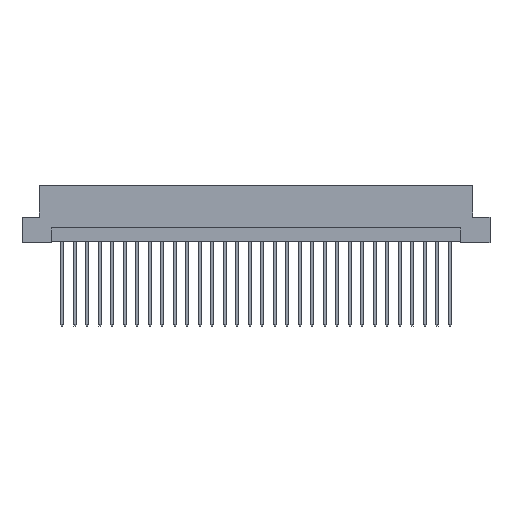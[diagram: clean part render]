
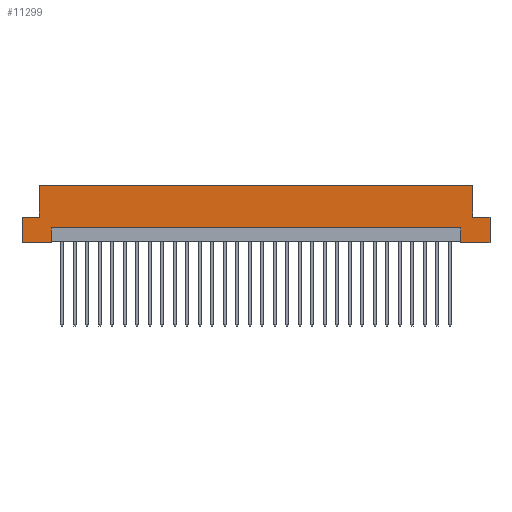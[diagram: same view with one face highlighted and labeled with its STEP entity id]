
A CAD part, front view. The second image highlights one B-rep face of the part: STEP entity #11299.
In plain terms, the highlighted planar face has unit normal (0, -1, 0).
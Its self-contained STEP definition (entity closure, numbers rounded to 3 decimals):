
#121 = VECTOR ( 'NONE', #6908, 1000. ) ;
#229 = VECTOR ( 'NONE', #6112, 1000. ) ;
#301 = DIRECTION ( 'NONE',  ( 0., 0., 1. ) ) ;
#396 = PLANE ( 'NONE',  #6061 ) ;
#691 = VERTEX_POINT ( 'NONE', #4877 ) ;
#767 = EDGE_CURVE ( 'NONE', #8356, #807, #3832, .T. ) ;
#798 = VECTOR ( 'NONE', #301, 1000. ) ;
#807 = VERTEX_POINT ( 'NONE', #4809 ) ;
#852 = CARTESIAN_POINT ( 'NONE',  ( -47.5, -4.3, 5.2 ) ) ;
#909 = CARTESIAN_POINT ( 'NONE',  ( -41.6, -4.3, 3. ) ) ;
#943 = ORIENTED_EDGE ( 'NONE', *, *, #10536, .T. ) ;
#1155 = CARTESIAN_POINT ( 'NONE',  ( 47.5, -4.3, 0. ) ) ;
#1309 = CARTESIAN_POINT ( 'NONE',  ( -47.5, -4.3, 0. ) ) ;
#1607 = LINE ( 'NONE', #7009, #10661 ) ;
#1705 = LINE ( 'NONE', #852, #11275 ) ;
#1811 = VERTEX_POINT ( 'NONE', #9847 ) ;
#1927 = DIRECTION ( 'NONE',  ( 1., 0., 0. ) ) ;
#2198 = LINE ( 'NONE', #10871, #5237 ) ;
#2203 = EDGE_CURVE ( 'NONE', #7240, #10167, #6225, .T. ) ;
#2415 = DIRECTION ( 'NONE',  ( 0., 1., 0. ) ) ;
#2458 = ORIENTED_EDGE ( 'NONE', *, *, #5085, .F. ) ;
#2568 = VERTEX_POINT ( 'NONE', #1309 ) ;
#2611 = CARTESIAN_POINT ( 'NONE',  ( -41.6, -4.3, 3. ) ) ;
#2728 = DIRECTION ( 'NONE',  ( 0., 0., -1. ) ) ;
#2834 = LINE ( 'NONE', #8767, #10973 ) ;
#2902 = ORIENTED_EDGE ( 'NONE', *, *, #3012, .F. ) ;
#2977 = VERTEX_POINT ( 'NONE', #5133 ) ;
#3012 = EDGE_CURVE ( 'NONE', #6895, #807, #11004, .T. ) ;
#3179 = DIRECTION ( 'NONE',  ( 1., 0., 0. ) ) ;
#3257 = CARTESIAN_POINT ( 'NONE',  ( 41.6, -4.3, 0. ) ) ;
#3782 = LINE ( 'NONE', #6784, #9607 ) ;
#3831 = CARTESIAN_POINT ( 'NONE',  ( -47.5, -4.3, 11.6 ) ) ;
#3832 = LINE ( 'NONE', #909, #11562 ) ;
#3837 = EDGE_CURVE ( 'NONE', #6895, #1811, #2834, .T. ) ;
#3967 = CARTESIAN_POINT ( 'NONE',  ( 47.5, -4.3, 11.6 ) ) ;
#4266 = ORIENTED_EDGE ( 'NONE', *, *, #2203, .T. ) ;
#4809 = CARTESIAN_POINT ( 'NONE',  ( 41.6, -4.3, 3. ) ) ;
#4877 = CARTESIAN_POINT ( 'NONE',  ( -47.5, -4.3, 5.2 ) ) ;
#5073 = CARTESIAN_POINT ( 'NONE',  ( 44., -4.3, 11.6 ) ) ;
#5085 = EDGE_CURVE ( 'NONE', #7240, #2977, #1607, .T. ) ;
#5127 = DIRECTION ( 'NONE',  ( 0., 0., -1. ) ) ;
#5133 = CARTESIAN_POINT ( 'NONE',  ( 47.5, -4.3, 5.2 ) ) ;
#5134 = CARTESIAN_POINT ( 'NONE',  ( 44., -4.3, 5.2 ) ) ;
#5237 = VECTOR ( 'NONE', #5127, 1000. ) ;
#5523 = CARTESIAN_POINT ( 'NONE',  ( -44., -4.3, 11.6 ) ) ;
#5667 = DIRECTION ( 'NONE',  ( 1., 0., 0. ) ) ;
#5680 = ORIENTED_EDGE ( 'NONE', *, *, #10644, .T. ) ;
#5845 = CARTESIAN_POINT ( 'NONE',  ( 47.5, -4.3, 11.6 ) ) ;
#6061 = AXIS2_PLACEMENT_3D ( 'NONE', #7374, #2415, #6393 ) ;
#6112 = DIRECTION ( 'NONE',  ( 1., 0., 0. ) ) ;
#6125 = EDGE_LOOP ( 'NONE', ( #11911, #2902, #8654, #11684, #2458, #4266, #11836, #9393, #7219, #943, #5680, #8408 ) ) ;
#6225 = LINE ( 'NONE', #10188, #798 ) ;
#6393 = DIRECTION ( 'NONE',  ( -1., 0., 0. ) ) ;
#6784 = CARTESIAN_POINT ( 'NONE',  ( -44., -4.3, 5.2 ) ) ;
#6895 = VERTEX_POINT ( 'NONE', #3257 ) ;
#6908 = DIRECTION ( 'NONE',  ( 0., 0., 1. ) ) ;
#7009 = CARTESIAN_POINT ( 'NONE',  ( 47.5, -4.3, 5.2 ) ) ;
#7219 = ORIENTED_EDGE ( 'NONE', *, *, #11336, .F. ) ;
#7240 = VERTEX_POINT ( 'NONE', #5134 ) ;
#7287 = EDGE_CURVE ( 'NONE', #8792, #10167, #9958, .T. ) ;
#7288 = VECTOR ( 'NONE', #3179, 1000. ) ;
#7374 = CARTESIAN_POINT ( 'NONE',  ( 47.5, -4.3, 11.6 ) ) ;
#7979 = CARTESIAN_POINT ( 'NONE',  ( -41.6, -4.3, 0. ) ) ;
#8356 = VERTEX_POINT ( 'NONE', #2611 ) ;
#8408 = ORIENTED_EDGE ( 'NONE', *, *, #11980, .F. ) ;
#8654 = ORIENTED_EDGE ( 'NONE', *, *, #3837, .T. ) ;
#8767 = CARTESIAN_POINT ( 'NONE',  ( 47.5, -4.3, 0. ) ) ;
#8792 = VERTEX_POINT ( 'NONE', #5523 ) ;
#8894 = VERTEX_POINT ( 'NONE', #10276 ) ;
#8933 = EDGE_CURVE ( 'NONE', #2977, #1811, #12662, .T. ) ;
#9172 = VECTOR ( 'NONE', #9563, 1000. ) ;
#9325 = FACE_OUTER_BOUND ( 'NONE', #6125, .T. ) ;
#9393 = ORIENTED_EDGE ( 'NONE', *, *, #11362, .F. ) ;
#9563 = DIRECTION ( 'NONE',  ( 0., 0., -1. ) ) ;
#9607 = VECTOR ( 'NONE', #11609, 1000. ) ;
#9829 = DIRECTION ( 'NONE',  ( 1., 0., 0. ) ) ;
#9847 = CARTESIAN_POINT ( 'NONE',  ( 47.5, -4.3, 0. ) ) ;
#9951 = LINE ( 'NONE', #1155, #229 ) ;
#9958 = LINE ( 'NONE', #3967, #7288 ) ;
#10167 = VERTEX_POINT ( 'NONE', #5073 ) ;
#10188 = CARTESIAN_POINT ( 'NONE',  ( 44., -4.3, 5.2 ) ) ;
#10276 = CARTESIAN_POINT ( 'NONE',  ( -44., -4.3, 5.2 ) ) ;
#10536 = EDGE_CURVE ( 'NONE', #691, #2568, #12805, .T. ) ;
#10644 = EDGE_CURVE ( 'NONE', #2568, #10915, #9951, .T. ) ;
#10661 = VECTOR ( 'NONE', #1927, 1000. ) ;
#10871 = CARTESIAN_POINT ( 'NONE',  ( -41.6, -4.3, 0.2 ) ) ;
#10915 = VERTEX_POINT ( 'NONE', #7979 ) ;
#10973 = VECTOR ( 'NONE', #11782, 1000. ) ;
#11004 = LINE ( 'NONE', #11879, #121 ) ;
#11275 = VECTOR ( 'NONE', #5667, 1000. ) ;
#11299 = ADVANCED_FACE ( 'NONE', ( #9325 ), #396, .F. ) ;
#11336 = EDGE_CURVE ( 'NONE', #691, #8894, #1705, .T. ) ;
#11362 = EDGE_CURVE ( 'NONE', #8894, #8792, #3782, .T. ) ;
#11469 = VECTOR ( 'NONE', #2728, 1000. ) ;
#11562 = VECTOR ( 'NONE', #9829, 1000. ) ;
#11609 = DIRECTION ( 'NONE',  ( 0., 0., 1. ) ) ;
#11684 = ORIENTED_EDGE ( 'NONE', *, *, #8933, .F. ) ;
#11782 = DIRECTION ( 'NONE',  ( 1., 0., 0. ) ) ;
#11836 = ORIENTED_EDGE ( 'NONE', *, *, #7287, .F. ) ;
#11879 = CARTESIAN_POINT ( 'NONE',  ( 41.6, -4.3, 0.2 ) ) ;
#11911 = ORIENTED_EDGE ( 'NONE', *, *, #767, .T. ) ;
#11980 = EDGE_CURVE ( 'NONE', #8356, #10915, #2198, .T. ) ;
#12662 = LINE ( 'NONE', #5845, #9172 ) ;
#12805 = LINE ( 'NONE', #3831, #11469 ) ;
